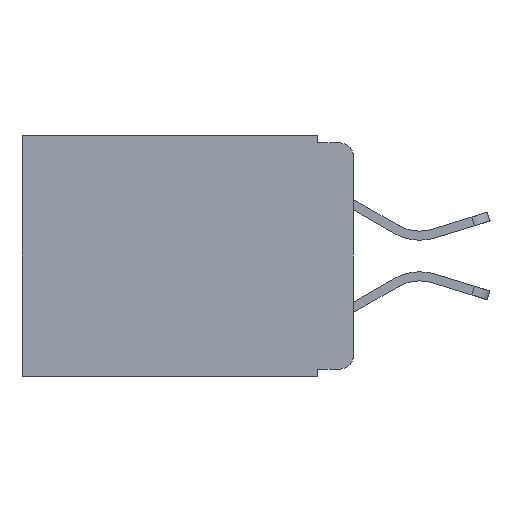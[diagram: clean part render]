
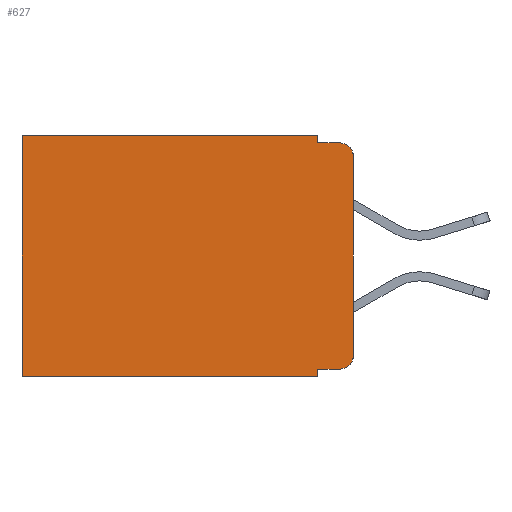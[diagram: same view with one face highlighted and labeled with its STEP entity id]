
A CAD part, left-side view. The second image highlights one B-rep face of the part: STEP entity #627.
In plain terms, the highlighted planar face has unit normal (-1, 0, 0).
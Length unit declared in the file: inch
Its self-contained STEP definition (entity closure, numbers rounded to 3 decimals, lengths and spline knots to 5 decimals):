
#627 = ADVANCED_FACE ( 'NONE', ( #8308 ), #13971, .F. ) ;
#684 = EDGE_CURVE ( 'NONE', #13700, #3734, #11150, .T. ) ;
#792 = CARTESIAN_POINT ( 'NONE',  ( 0.298, 0.02, -0.03 ) ) ;
#1096 = LINE ( 'NONE', #1462, #4147 ) ;
#1111 = VERTEX_POINT ( 'NONE', #16120 ) ;
#1226 = EDGE_CURVE ( 'NONE', #5323, #7505, #6708, .T. ) ;
#1228 = ORIENTED_EDGE ( 'NONE', *, *, #684, .T. ) ;
#1319 = VERTEX_POINT ( 'NONE', #9022 ) ;
#1432 = AXIS2_PLACEMENT_3D ( 'NONE', #6657, #10873, #9777 ) ;
#1462 = CARTESIAN_POINT ( 'NONE',  ( 0.298, 0., 0. ) ) ;
#1710 = CARTESIAN_POINT ( 'NONE',  ( 0.298, 0.473, 0. ) ) ;
#1882 = VERTEX_POINT ( 'NONE', #16164 ) ;
#1895 = VECTOR ( 'NONE', #4446, 39.37008 ) ;
#1904 = CARTESIAN_POINT ( 'NONE',  ( 0.298, 0.02, -0.313 ) ) ;
#2346 = LINE ( 'NONE', #14263, #1895 ) ;
#2537 = CARTESIAN_POINT ( 'NONE',  ( 0.298, 0.02, -0.333 ) ) ;
#2997 = CARTESIAN_POINT ( 'NONE',  ( 0.298, 0.051, -0.01 ) ) ;
#3164 = CARTESIAN_POINT ( 'NONE',  ( 0.298, 0.051, -0.01 ) ) ;
#3244 = DIRECTION ( 'NONE',  ( 0., 0., -1. ) ) ;
#3460 = EDGE_CURVE ( 'NONE', #15816, #7505, #11726, .T. ) ;
#3597 = CARTESIAN_POINT ( 'NONE',  ( 0.298, 0.02, -0.01 ) ) ;
#3734 = VERTEX_POINT ( 'NONE', #6492 ) ;
#3830 = ORIENTED_EDGE ( 'NONE', *, *, #1226, .F. ) ;
#3943 = EDGE_CURVE ( 'NONE', #1882, #15749, #1096, .T. ) ;
#4147 = VECTOR ( 'NONE', #17394, 39.37008 ) ;
#4446 = DIRECTION ( 'NONE',  ( 0., 0., -1. ) ) ;
#4488 = CARTESIAN_POINT ( 'NONE',  ( 0.298, 0.051, -0.333 ) ) ;
#5073 = VECTOR ( 'NONE', #7339, 39.37008 ) ;
#5323 = VERTEX_POINT ( 'NONE', #2997 ) ;
#5397 = ORIENTED_EDGE ( 'NONE', *, *, #14754, .F. ) ;
#5417 = ORIENTED_EDGE ( 'NONE', *, *, #9060, .T. ) ;
#5566 = VECTOR ( 'NONE', #8094, 39.37008 ) ;
#5933 = DIRECTION ( 'NONE',  ( 0., -1., 0. ) ) ;
#6355 = AXIS2_PLACEMENT_3D ( 'NONE', #1904, #14529, #14287 ) ;
#6492 = CARTESIAN_POINT ( 'NONE',  ( 0.298, 0., -0.313 ) ) ;
#6578 = CARTESIAN_POINT ( 'NONE',  ( 0.298, 0., 0. ) ) ;
#6626 = AXIS2_PLACEMENT_3D ( 'NONE', #792, #12081, #3244 ) ;
#6657 = CARTESIAN_POINT ( 'NONE',  ( 0.298, 0., 0. ) ) ;
#6708 = LINE ( 'NONE', #3164, #13296 ) ;
#6969 = ORIENTED_EDGE ( 'NONE', *, *, #11479, .F. ) ;
#7339 = DIRECTION ( 'NONE',  ( 0., 0., -1. ) ) ;
#7437 = VECTOR ( 'NONE', #5933, 39.37008 ) ;
#7505 = VERTEX_POINT ( 'NONE', #3597 ) ;
#7877 = EDGE_CURVE ( 'NONE', #8024, #1319, #2346, .T. ) ;
#7900 = LINE ( 'NONE', #4488, #7437 ) ;
#8024 = VERTEX_POINT ( 'NONE', #10681 ) ;
#8094 = DIRECTION ( 'NONE',  ( 0., 0., -1. ) ) ;
#8109 = EDGE_CURVE ( 'NONE', #1882, #5323, #13040, .T. ) ;
#8113 = ORIENTED_EDGE ( 'NONE', *, *, #16278, .T. ) ;
#8308 = FACE_OUTER_BOUND ( 'NONE', #10874, .T. ) ;
#9022 = CARTESIAN_POINT ( 'NONE',  ( 0.298, 0.051, -0.343 ) ) ;
#9060 = EDGE_CURVE ( 'NONE', #15749, #1111, #12155, .T. ) ;
#9309 = DIRECTION ( 'NONE',  ( 0., 1., 0. ) ) ;
#9699 = VECTOR ( 'NONE', #14917, 39.37008 ) ;
#9777 = DIRECTION ( 'NONE',  ( 0., 0., -1. ) ) ;
#10079 = DIRECTION ( 'NONE',  ( 0., -1., 0. ) ) ;
#10554 = CARTESIAN_POINT ( 'NONE',  ( 0.298, 0., -0.03 ) ) ;
#10681 = CARTESIAN_POINT ( 'NONE',  ( 0.298, 0.051, -0.333 ) ) ;
#10873 = DIRECTION ( 'NONE',  ( 1., 0., 0. ) ) ;
#10874 = EDGE_LOOP ( 'NONE', ( #6969, #13119, #3830, #16943, #17581, #5417, #5397, #13529, #8113, #1228 ) ) ;
#11150 = CIRCLE ( 'NONE', #6355, 0.02 ) ;
#11479 = EDGE_CURVE ( 'NONE', #15816, #3734, #13355, .T. ) ;
#11668 = LINE ( 'NONE', #13390, #18054 ) ;
#11726 = CIRCLE ( 'NONE', #6626, 0.02 ) ;
#12081 = DIRECTION ( 'NONE',  ( -1., 0., 0. ) ) ;
#12155 = LINE ( 'NONE', #14347, #5073 ) ;
#13040 = LINE ( 'NONE', #17714, #5566 ) ;
#13119 = ORIENTED_EDGE ( 'NONE', *, *, #3460, .T. ) ;
#13296 = VECTOR ( 'NONE', #10079, 39.37008 ) ;
#13355 = LINE ( 'NONE', #6578, #9699 ) ;
#13390 = CARTESIAN_POINT ( 'NONE',  ( 0.298, 0., -0.343 ) ) ;
#13529 = ORIENTED_EDGE ( 'NONE', *, *, #7877, .F. ) ;
#13700 = VERTEX_POINT ( 'NONE', #2537 ) ;
#13971 = PLANE ( 'NONE',  #1432 ) ;
#14263 = CARTESIAN_POINT ( 'NONE',  ( 0.298, 0.051, 0. ) ) ;
#14287 = DIRECTION ( 'NONE',  ( 0., 0., -1. ) ) ;
#14347 = CARTESIAN_POINT ( 'NONE',  ( 0.298, 0.473, 0. ) ) ;
#14529 = DIRECTION ( 'NONE',  ( -1., 0., 0. ) ) ;
#14754 = EDGE_CURVE ( 'NONE', #1319, #1111, #11668, .T. ) ;
#14917 = DIRECTION ( 'NONE',  ( 0., 0., -1. ) ) ;
#15749 = VERTEX_POINT ( 'NONE', #1710 ) ;
#15816 = VERTEX_POINT ( 'NONE', #10554 ) ;
#16120 = CARTESIAN_POINT ( 'NONE',  ( 0.298, 0.473, -0.343 ) ) ;
#16164 = CARTESIAN_POINT ( 'NONE',  ( 0.298, 0.051, 0. ) ) ;
#16278 = EDGE_CURVE ( 'NONE', #8024, #13700, #7900, .T. ) ;
#16943 = ORIENTED_EDGE ( 'NONE', *, *, #8109, .F. ) ;
#17394 = DIRECTION ( 'NONE',  ( 0., 1., 0. ) ) ;
#17581 = ORIENTED_EDGE ( 'NONE', *, *, #3943, .T. ) ;
#17714 = CARTESIAN_POINT ( 'NONE',  ( 0.298, 0.051, 0. ) ) ;
#18054 = VECTOR ( 'NONE', #9309, 39.37008 ) ;
